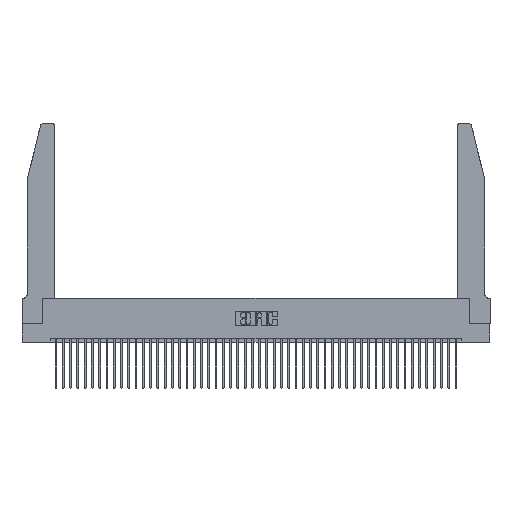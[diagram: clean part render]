
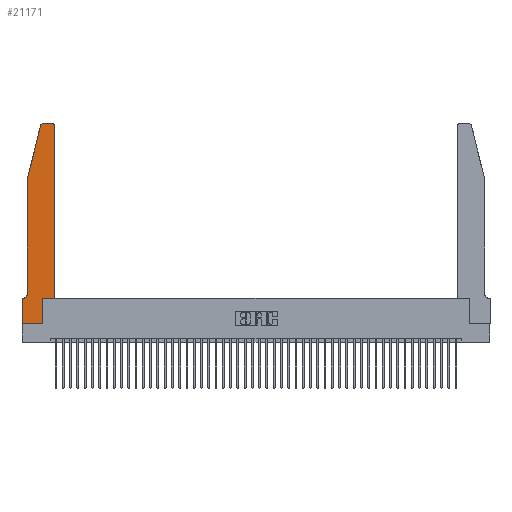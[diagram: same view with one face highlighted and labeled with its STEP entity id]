
A CAD part, top view. The second image highlights one B-rep face of the part: STEP entity #21171.
In plain terms, the highlighted planar face has unit normal (0, 0, 1).
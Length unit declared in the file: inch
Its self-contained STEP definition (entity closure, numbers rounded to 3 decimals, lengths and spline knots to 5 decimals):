
#912 = LINE ( 'NONE', #16278, #29912 ) ;
#1102 = DIRECTION ( 'NONE',  ( 0., -1., 0. ) ) ;
#1416 = ORIENTED_EDGE ( 'NONE', *, *, #38017, .T. ) ;
#1624 = VERTEX_POINT ( 'NONE', #15919 ) ;
#1717 = ORIENTED_EDGE ( 'NONE', *, *, #45506, .T. ) ;
#2718 = CIRCLE ( 'NONE', #12304, 0.03 ) ;
#2808 = LINE ( 'NONE', #33639, #29473 ) ;
#3144 = VECTOR ( 'NONE', #6517, 39.37008 ) ;
#3394 = DIRECTION ( 'NONE',  ( 0., 1., 0. ) ) ;
#3476 = CARTESIAN_POINT ( 'NONE',  ( 0.4205, 2.75, 0.37 ) ) ;
#3801 = DIRECTION ( 'NONE',  ( -1., 0., 0. ) ) ;
#4135 = CARTESIAN_POINT ( 'NONE',  ( 0., 0.35, 0.37 ) ) ;
#5803 = VERTEX_POINT ( 'NONE', #12391 ) ;
#5953 = EDGE_CURVE ( 'NONE', #28234, #46557, #28304, .T. ) ;
#6234 = EDGE_CURVE ( 'NONE', #27663, #8957, #26547, .T. ) ;
#6517 = DIRECTION ( 'NONE',  ( -1., 0., 0. ) ) ;
#6692 = VECTOR ( 'NONE', #18587, 39.37008 ) ;
#6701 = FACE_OUTER_BOUND ( 'NONE', #20625, .T. ) ;
#7785 = DIRECTION ( 'NONE',  ( 1., 0., 0. ) ) ;
#7797 = EDGE_CURVE ( 'NONE', #1624, #45391, #912, .T. ) ;
#8826 = AXIS2_PLACEMENT_3D ( 'NONE', #10715, #36047, #14339 ) ;
#8842 = ORIENTED_EDGE ( 'NONE', *, *, #44001, .T. ) ;
#8957 = VERTEX_POINT ( 'NONE', #33909 ) ;
#9047 = ORIENTED_EDGE ( 'NONE', *, *, #24050, .T. ) ;
#10262 = CARTESIAN_POINT ( 'NONE',  ( 0.2865, 0., 0.37 ) ) ;
#10350 = CARTESIAN_POINT ( 'NONE',  ( 0.25487, 2.72718, 0.37 ) ) ;
#10692 = CARTESIAN_POINT ( 'NONE',  ( 0.0755, 2., 0.37 ) ) ;
#10715 = CARTESIAN_POINT ( 'NONE',  ( 0.284, 2.72, 0.37 ) ) ;
#11006 = EDGE_CURVE ( 'NONE', #12121, #20960, #34191, .T. ) ;
#11652 = LINE ( 'NONE', #28186, #3144 ) ;
#11756 = ORIENTED_EDGE ( 'NONE', *, *, #46036, .T. ) ;
#12121 = VERTEX_POINT ( 'NONE', #39090 ) ;
#12304 = AXIS2_PLACEMENT_3D ( 'NONE', #40901, #19286, #44504 ) ;
#12391 = CARTESIAN_POINT ( 'NONE',  ( 0.4505, 2.72, 0.37 ) ) ;
#12809 = CARTESIAN_POINT ( 'NONE',  ( 0.0755, 0.42, 0.37 ) ) ;
#13285 = CARTESIAN_POINT ( 'NONE',  ( 0., 0., 0.37 ) ) ;
#14339 = DIRECTION ( 'NONE',  ( 1., 0., 0. ) ) ;
#15919 = CARTESIAN_POINT ( 'NONE',  ( 0.2865, 0.35, 0.37 ) ) ;
#16278 = CARTESIAN_POINT ( 'NONE',  ( 0.4505, 0.35, 0.37 ) ) ;
#16394 = DIRECTION ( 'NONE',  ( -0.239, -0.971, 0. ) ) ;
#17310 = VECTOR ( 'NONE', #3394, 39.37008 ) ;
#17851 = CARTESIAN_POINT ( 'NONE',  ( 0.4505, 0.35, 0.37 ) ) ;
#18587 = DIRECTION ( 'NONE',  ( 0., -1., 0. ) ) ;
#18660 = VECTOR ( 'NONE', #42119, 39.37008 ) ;
#19255 = DIRECTION ( 'NONE',  ( 0., 0., -1. ) ) ;
#19286 = DIRECTION ( 'NONE',  ( 0., 0., 1. ) ) ;
#20506 = CARTESIAN_POINT ( 'NONE',  ( 0., 0., 0.37 ) ) ;
#20625 = EDGE_LOOP ( 'NONE', ( #1717, #39567, #11756, #46265, #9047, #22999, #33252, #39970, #37007, #41036, #1416, #8842 ) ) ;
#20673 = DIRECTION ( 'NONE',  ( 0., 1., 0. ) ) ;
#20960 = VERTEX_POINT ( 'NONE', #10350 ) ;
#20991 = CIRCLE ( 'NONE', #22244, 0.07 ) ;
#21171 = ADVANCED_FACE ( 'NONE', ( #6701 ), #40173, .T. ) ;
#22244 = AXIS2_PLACEMENT_3D ( 'NONE', #40875, #19255, #44481 ) ;
#22999 = ORIENTED_EDGE ( 'NONE', *, *, #6234, .T. ) ;
#23169 = VECTOR ( 'NONE', #20673, 39.37008 ) ;
#24050 = EDGE_CURVE ( 'NONE', #43485, #27663, #20991, .T. ) ;
#24059 = EDGE_CURVE ( 'NONE', #8957, #28234, #2808, .T. ) ;
#25432 = VECTOR ( 'NONE', #3801, 39.37008 ) ;
#26547 = LINE ( 'NONE', #32778, #25432 ) ;
#27663 = VERTEX_POINT ( 'NONE', #28236 ) ;
#28077 = LINE ( 'NONE', #17851, #17310 ) ;
#28186 = CARTESIAN_POINT ( 'NONE',  ( 0.2605, 2.75, 0.37 ) ) ;
#28234 = VERTEX_POINT ( 'NONE', #13285 ) ;
#28236 = CARTESIAN_POINT ( 'NONE',  ( 0.0055, 0.35, 0.37 ) ) ;
#28304 = LINE ( 'NONE', #20506, #18660 ) ;
#29473 = VECTOR ( 'NONE', #1102, 39.37008 ) ;
#29483 = DIRECTION ( 'NONE',  ( 0., 0., 1. ) ) ;
#29912 = VECTOR ( 'NONE', #37960, 39.37008 ) ;
#30846 = CARTESIAN_POINT ( 'NONE',  ( 0.0755, 2., 0.37 ) ) ;
#32778 = CARTESIAN_POINT ( 'NONE',  ( 0.0755, 0.35, 0.37 ) ) ;
#33252 = ORIENTED_EDGE ( 'NONE', *, *, #24059, .T. ) ;
#33639 = CARTESIAN_POINT ( 'NONE',  ( 0., 0., 0.37 ) ) ;
#33909 = CARTESIAN_POINT ( 'NONE',  ( 0., 0.35, 0.37 ) ) ;
#34191 = CIRCLE ( 'NONE', #8826, 0.03 ) ;
#34483 = EDGE_CURVE ( 'NONE', #46557, #1624, #42379, .T. ) ;
#36047 = DIRECTION ( 'NONE',  ( 0., 0., 1. ) ) ;
#36623 = CARTESIAN_POINT ( 'NONE',  ( 0.0755, 2., 0.37 ) ) ;
#36655 = EDGE_CURVE ( 'NONE', #42084, #43485, #46670, .T. ) ;
#37007 = ORIENTED_EDGE ( 'NONE', *, *, #34483, .T. ) ;
#37099 = VECTOR ( 'NONE', #16394, 39.37008 ) ;
#37960 = DIRECTION ( 'NONE',  ( 1., 0., 0. ) ) ;
#38017 = EDGE_CURVE ( 'NONE', #45391, #5803, #28077, .T. ) ;
#38650 = CARTESIAN_POINT ( 'NONE',  ( 0.2865, 0.35, 0.37 ) ) ;
#39090 = CARTESIAN_POINT ( 'NONE',  ( 0.284, 2.75, 0.37 ) ) ;
#39567 = ORIENTED_EDGE ( 'NONE', *, *, #11006, .T. ) ;
#39970 = ORIENTED_EDGE ( 'NONE', *, *, #5953, .T. ) ;
#40173 = PLANE ( 'NONE',  #41528 ) ;
#40875 = CARTESIAN_POINT ( 'NONE',  ( 0.0055, 0.42, 0.37 ) ) ;
#40901 = CARTESIAN_POINT ( 'NONE',  ( 0.4205, 2.72, 0.37 ) ) ;
#41036 = ORIENTED_EDGE ( 'NONE', *, *, #7797, .T. ) ;
#41528 = AXIS2_PLACEMENT_3D ( 'NONE', #4135, #29483, #7785 ) ;
#41895 = CARTESIAN_POINT ( 'NONE',  ( 0.4505, 0.35, 0.37 ) ) ;
#42084 = VERTEX_POINT ( 'NONE', #10692 ) ;
#42119 = DIRECTION ( 'NONE',  ( 1., 0., 0. ) ) ;
#42379 = LINE ( 'NONE', #38650, #23169 ) ;
#42778 = VERTEX_POINT ( 'NONE', #3476 ) ;
#43485 = VERTEX_POINT ( 'NONE', #12809 ) ;
#44001 = EDGE_CURVE ( 'NONE', #5803, #42778, #2718, .T. ) ;
#44481 = DIRECTION ( 'NONE',  ( -1., 0., 0. ) ) ;
#44504 = DIRECTION ( 'NONE',  ( 1., 0., 0. ) ) ;
#45391 = VERTEX_POINT ( 'NONE', #41895 ) ;
#45492 = LINE ( 'NONE', #30846, #37099 ) ;
#45506 = EDGE_CURVE ( 'NONE', #42778, #12121, #11652, .T. ) ;
#46036 = EDGE_CURVE ( 'NONE', #20960, #42084, #45492, .T. ) ;
#46265 = ORIENTED_EDGE ( 'NONE', *, *, #36655, .T. ) ;
#46557 = VERTEX_POINT ( 'NONE', #10262 ) ;
#46670 = LINE ( 'NONE', #36623, #6692 ) ;
